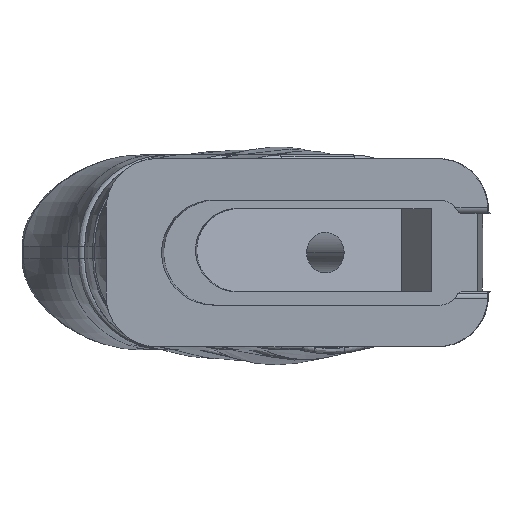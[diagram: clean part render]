
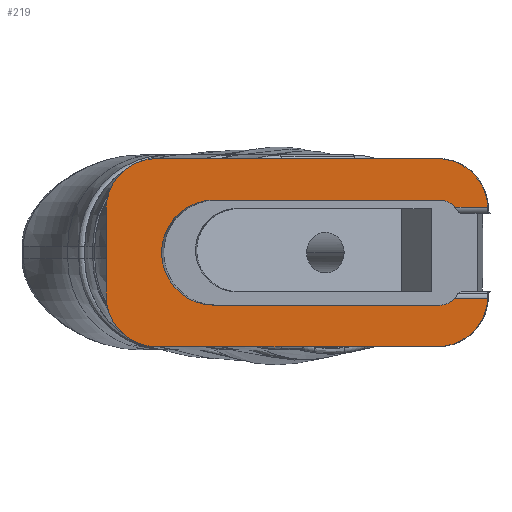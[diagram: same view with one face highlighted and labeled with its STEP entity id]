
A CAD part, front view. The second image highlights one B-rep face of the part: STEP entity #219.
In plain terms, the highlighted face is planar.
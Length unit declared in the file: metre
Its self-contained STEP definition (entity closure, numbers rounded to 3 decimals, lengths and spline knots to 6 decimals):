
#219=ADVANCED_FACE('14:448251',(#1280),#1281,.F.);
#1280=FACE_OUTER_BOUND('',#3225,.T.);
#1281=PLANE('',#3226);
#3225=EDGE_LOOP('',(#66170,#66171,#66172,#66173,#66174,#66175,#66176,#66177,#66178,#66179,#66180,#66181,#66182,#66183,#66184));
#3226=AXIS2_PLACEMENT_3D('',#66185,#66186,#66187);
#66170=ORIENTED_EDGE('',*,*,#74126,.T.);
#66171=ORIENTED_EDGE('',*,*,#74127,.T.);
#66172=ORIENTED_EDGE('',*,*,#74128,.T.);
#66173=ORIENTED_EDGE('',*,*,#74129,.T.);
#66174=ORIENTED_EDGE('',*,*,#74130,.T.);
#66175=ORIENTED_EDGE('',*,*,#74131,.T.);
#66176=ORIENTED_EDGE('',*,*,#74132,.F.);
#66177=ORIENTED_EDGE('',*,*,#74133,.F.);
#66178=ORIENTED_EDGE('',*,*,#74134,.F.);
#66179=ORIENTED_EDGE('',*,*,#74135,.F.);
#66180=ORIENTED_EDGE('',*,*,#73802,.F.);
#66181=ORIENTED_EDGE('',*,*,#74136,.F.);
#66182=ORIENTED_EDGE('',*,*,#74124,.T.);
#66183=ORIENTED_EDGE('',*,*,#74105,.F.);
#66184=ORIENTED_EDGE('',*,*,#74109,.F.);
#66185=CARTESIAN_POINT('',(-0.147412,-0.2448,0.167681));
#66186=DIRECTION('',(-0.06,0.,-0.998));
#66187=DIRECTION('',(0.,1.0,0.));
#73802=EDGE_CURVE('10:7170',#76411,#76413,#76414,.T.);
#74105=EDGE_CURVE('14:448278',#77007,#77009,#77010,.T.);
#74109=EDGE_CURVE('10:7257',#77014,#77007,#77016,.T.);
#74124=EDGE_CURVE('10:7245',#77044,#77009,#77045,.T.);
#74126=EDGE_CURVE('10:7215',#77014,#77047,#77048,.T.);
#74127=EDGE_CURVE('10:7218',#77047,#77049,#77050,.T.);
#74128=EDGE_CURVE('10:7221',#77049,#77051,#77052,.T.);
#74129=EDGE_CURVE('12:48363',#77051,#77053,#77054,.T.);
#74130=EDGE_CURVE('10:7227',#77053,#77055,#77056,.T.);
#74131=EDGE_CURVE('10:7230',#77055,#77057,#77058,.T.);
#74132=EDGE_CURVE('10:7233',#77059,#77057,#77060,.T.);
#74133=EDGE_CURVE('10:7236',#77061,#77059,#77062,.T.);
#74134=EDGE_CURVE('10:7239',#77063,#77061,#77064,.T.);
#74135=EDGE_CURVE('12:47817',#76413,#77063,#77065,.T.);
#74136=EDGE_CURVE('10:7242',#77044,#76411,#77066,.T.);
#76411=VERTEX_POINT('',#80816);
#76413=VERTEX_POINT('',#80821);
#76414=LINE('',#80822,#80823);
#77007=VERTEX_POINT('',#82565);
#77009=VERTEX_POINT('',#82568);
#77010=CIRCLE('',#82569,0.008295);
#77014=VERTEX_POINT('',#82575);
#77016=LINE('',#82578,#82579);
#77044=VERTEX_POINT('',#82616);
#77045=LINE('',#82617,#82618);
#77047=VERTEX_POINT('',#82621);
#77048=CIRCLE('',#82622,0.003);
#77049=VERTEX_POINT('',#82623);
#77050=LINE('',#82624,#82625);
#77051=VERTEX_POINT('',#82626);
#77052=LINE('',#82627,#82628);
#77053=VERTEX_POINT('',#82629);
#77054=CIRCLE('',#82630,0.008);
#77055=VERTEX_POINT('',#82631);
#77056=LINE('',#82632,#82633);
#77057=VERTEX_POINT('',#82634);
#77058=CIRCLE('',#82635,0.008);
#77059=VERTEX_POINT('',#82636);
#77060=LINE('',#82637,#82638);
#77061=VERTEX_POINT('',#82639);
#77062=CIRCLE('',#82640,0.008);
#77063=VERTEX_POINT('',#82641);
#77064=LINE('',#82642,#82643);
#77065=CIRCLE('',#82644,0.008);
#77066=CIRCLE('',#82645,0.003);
#80816=CARTESIAN_POINT('',(-0.152626,-0.237125,0.167996));
#80821=CARTESIAN_POINT('',(-0.147418,-0.237125,0.167681));
#80822=CARTESIAN_POINT('',(-0.147412,-0.237125,0.167681));
#80823=VECTOR('',#99934,1.0);
#82565=CARTESIAN_POINT('',(-0.190585,-0.221655,0.17029));
#82568=CARTESIAN_POINT('',(-0.190585,-0.238246,0.17029));
#82569=AXIS2_PLACEMENT_3D('',#100437,#100438,#100439);
#82575=CARTESIAN_POINT('',(-0.15496,-0.221655,0.168137));
#82578=CARTESIAN_POINT('',(-0.15041,-0.221655,0.167862));
#82579=VECTOR('',#100443,1.0);
#82616=CARTESIAN_POINT('',(-0.15496,-0.238246,0.168137));
#82617=CARTESIAN_POINT('',(-0.15041,-0.238246,0.167862));
#82618=VECTOR('',#100468,1.0);
#82621=CARTESIAN_POINT('',(-0.152514,-0.222924,0.167989));
#82622=AXIS2_PLACEMENT_3D('',#100470,#100471,#100472);
#82623=CARTESIAN_POINT('',(-0.152619,-0.222775,0.167996));
#82624=CARTESIAN_POINT('',(-0.146219,-0.231851,0.167609));
#82625=VECTOR('',#100473,1.0);
#82626=CARTESIAN_POINT('',(-0.147418,-0.222775,0.167681));
#82627=CARTESIAN_POINT('',(-0.147412,-0.222775,0.167681));
#82628=VECTOR('',#100474,1.0);
#82629=CARTESIAN_POINT('',(-0.155397,-0.2151,0.168164));
#82630=AXIS2_PLACEMENT_3D('',#100475,#100476,#100477);
#82631=CARTESIAN_POINT('',(-0.199606,-0.2151,0.170835));
#82632=CARTESIAN_POINT('',(-0.155397,-0.2151,0.168164));
#82633=VECTOR('',#100478,0.04429);
#82634=CARTESIAN_POINT('',(-0.207592,-0.2231,0.171317));
#82635=AXIS2_PLACEMENT_3D('',#100479,#100480,#100481);
#82636=CARTESIAN_POINT('',(-0.207592,-0.2368,0.171317));
#82637=CARTESIAN_POINT('',(-0.207592,-0.236075,0.171317));
#82638=VECTOR('',#100482,0.01225);
#82639=CARTESIAN_POINT('',(-0.199606,-0.2448,0.170835));
#82640=AXIS2_PLACEMENT_3D('',#100483,#100484,#100485);
#82641=CARTESIAN_POINT('',(-0.155397,-0.2448,0.168164));
#82642=CARTESIAN_POINT('',(-0.155397,-0.2448,0.168164));
#82643=VECTOR('',#100486,0.04429);
#82644=AXIS2_PLACEMENT_3D('',#100487,#100488,#100489);
#82645=AXIS2_PLACEMENT_3D('',#100490,#100491,#100492);
#99934=DIRECTION('',(0.998,0.,-0.06));
#100437=CARTESIAN_POINT('',(-0.190585,-0.22995,0.17029));
#100438=DIRECTION('',(0.06,0.,0.998));
#100439=DIRECTION('',(0.,-1.0,0.));
#100443=DIRECTION('',(-0.998,0.,0.06));
#100468=DIRECTION('',(-0.998,0.,0.06));
#100470=CARTESIAN_POINT('',(-0.15496,-0.224655,0.168137));
#100471=DIRECTION('',(-0.06,0.,-0.998));
#100472=DIRECTION('',(0.,1.0,0.));
#100473=DIRECTION('',(-0.576,0.817,0.035));
#100474=DIRECTION('',(0.998,0.,-0.06));
#100475=CARTESIAN_POINT('',(-0.155397,-0.2231,0.168164));
#100476=DIRECTION('',(0.06,0.,0.998));
#100477=DIRECTION('',(0.,1.0,0.));
#100478=DIRECTION('',(-0.998,0.,0.06));
#100479=CARTESIAN_POINT('',(-0.199606,-0.2231,0.170835));
#100480=DIRECTION('',(0.06,0.,0.998));
#100481=DIRECTION('',(0.,-1.0,0.));
#100482=DIRECTION('',(0.,1.0,0.));
#100483=CARTESIAN_POINT('',(-0.199606,-0.2368,0.170835));
#100484=DIRECTION('',(-0.06,0.,-0.998));
#100485=DIRECTION('',(0.,1.0,0.));
#100486=DIRECTION('',(-0.998,0.,0.06));
#100487=CARTESIAN_POINT('',(-0.155397,-0.2368,0.168164));
#100488=DIRECTION('',(-0.06,0.,-0.998));
#100489=DIRECTION('',(0.,-1.0,0.));
#100490=CARTESIAN_POINT('',(-0.15496,-0.235246,0.168137));
#100491=DIRECTION('',(0.06,0.,0.998));
#100492=DIRECTION('',(0.,-1.0,0.));
